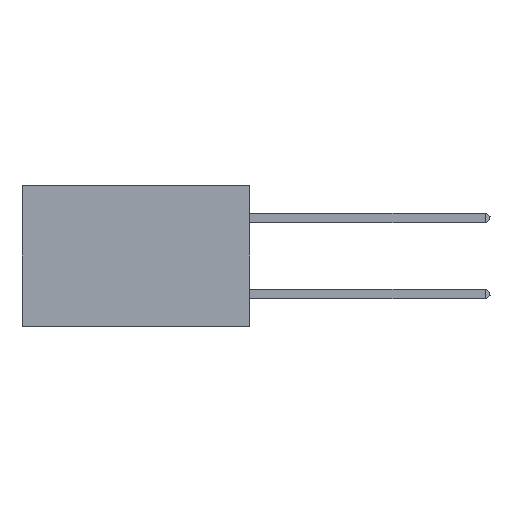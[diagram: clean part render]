
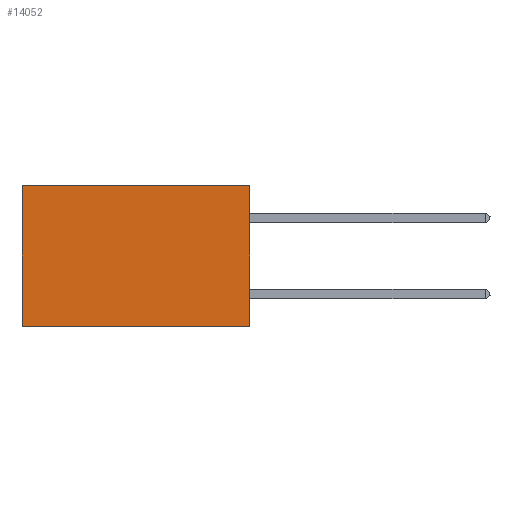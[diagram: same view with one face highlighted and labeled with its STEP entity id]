
A CAD part, left-side view. The second image highlights one B-rep face of the part: STEP entity #14052.
In plain terms, the highlighted planar face has unit normal (-1, 0, 0).
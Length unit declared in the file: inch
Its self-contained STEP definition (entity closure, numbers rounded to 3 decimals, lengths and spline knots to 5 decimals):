
#6 = CARTESIAN_POINT ( 'NONE',  ( 0.2875, 0., 0. ) ) ;
#371 = DIRECTION ( 'NONE',  ( 0., 1., 0. ) ) ;
#690 = LINE ( 'NONE', #25289, #27878 ) ;
#2761 = DIRECTION ( 'NONE',  ( 0., 0., -1. ) ) ;
#3896 = CARTESIAN_POINT ( 'NONE',  ( 0.2875, 0.6, -0.37 ) ) ;
#4373 = EDGE_CURVE ( 'NONE', #7179, #16298, #690, .T. ) ;
#7179 = VERTEX_POINT ( 'NONE', #26586 ) ;
#7240 = EDGE_CURVE ( 'NONE', #16298, #30568, #17177, .T. ) ;
#10001 = LINE ( 'NONE', #17317, #23133 ) ;
#10542 = CARTESIAN_POINT ( 'NONE',  ( 0.2875, 0., -0.37 ) ) ;
#11478 = VECTOR ( 'NONE', #27931, 39.37008 ) ;
#12292 = CARTESIAN_POINT ( 'NONE',  ( 0.2875, 0., -0.37 ) ) ;
#13713 = DIRECTION ( 'NONE',  ( 0., 0., -1. ) ) ;
#14052 = ADVANCED_FACE ( 'NONE', ( #23612 ), #23573, .F. ) ;
#14252 = AXIS2_PLACEMENT_3D ( 'NONE', #6, #18602, #2761 ) ;
#15833 = ORIENTED_EDGE ( 'NONE', *, *, #7240, .T. ) ;
#16227 = EDGE_CURVE ( 'NONE', #16519, #30568, #31501, .T. ) ;
#16298 = VERTEX_POINT ( 'NONE', #33360 ) ;
#16519 = VERTEX_POINT ( 'NONE', #10542 ) ;
#17177 = LINE ( 'NONE', #26811, #24888 ) ;
#17271 = EDGE_LOOP ( 'NONE', ( #15833, #18948, #30343, #26836 ) ) ;
#17317 = CARTESIAN_POINT ( 'NONE',  ( 0.2875, 0., 0. ) ) ;
#18602 = DIRECTION ( 'NONE',  ( 1., 0., 0. ) ) ;
#18948 = ORIENTED_EDGE ( 'NONE', *, *, #16227, .F. ) ;
#23133 = VECTOR ( 'NONE', #32952, 39.37008 ) ;
#23573 = PLANE ( 'NONE',  #14252 ) ;
#23612 = FACE_OUTER_BOUND ( 'NONE', #17271, .T. ) ;
#24888 = VECTOR ( 'NONE', #13713, 39.37008 ) ;
#25289 = CARTESIAN_POINT ( 'NONE',  ( 0.2875, 0., 0. ) ) ;
#26586 = CARTESIAN_POINT ( 'NONE',  ( 0.2875, 0., 0. ) ) ;
#26811 = CARTESIAN_POINT ( 'NONE',  ( 0.2875, 0.6, 0. ) ) ;
#26836 = ORIENTED_EDGE ( 'NONE', *, *, #4373, .T. ) ;
#27878 = VECTOR ( 'NONE', #371, 39.37008 ) ;
#27931 = DIRECTION ( 'NONE',  ( 0., 1., 0. ) ) ;
#28664 = EDGE_CURVE ( 'NONE', #7179, #16519, #10001, .T. ) ;
#30343 = ORIENTED_EDGE ( 'NONE', *, *, #28664, .F. ) ;
#30568 = VERTEX_POINT ( 'NONE', #3896 ) ;
#31501 = LINE ( 'NONE', #12292, #11478 ) ;
#32952 = DIRECTION ( 'NONE',  ( 0., 0., -1. ) ) ;
#33360 = CARTESIAN_POINT ( 'NONE',  ( 0.2875, 0.6, 0. ) ) ;
